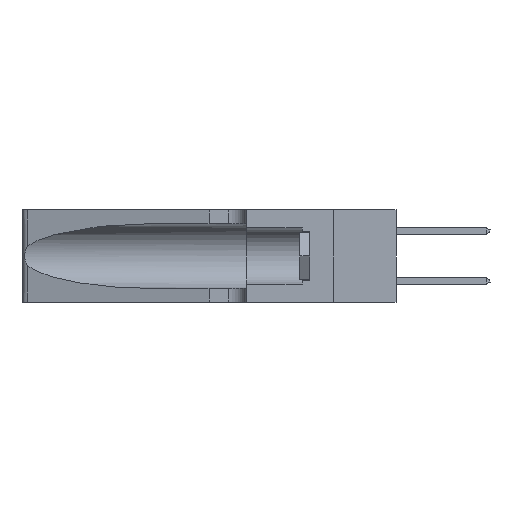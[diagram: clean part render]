
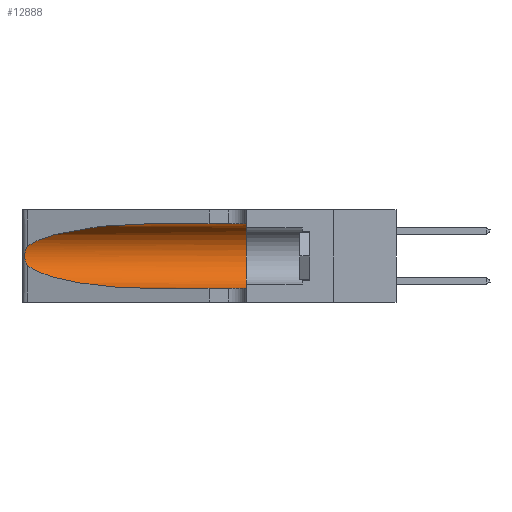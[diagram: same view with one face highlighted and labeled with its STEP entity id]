
A CAD part, left-side view. The second image highlights one B-rep face of the part: STEP entity #12888.
In plain terms, the highlighted cylindrical face has radius 3.308 mm (diameter 6.617 mm), a partial arc.
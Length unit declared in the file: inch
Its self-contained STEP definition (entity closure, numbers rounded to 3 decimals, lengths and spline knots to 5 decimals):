
#367 = AXIS2_PLACEMENT_3D ( 'NONE', #13925, #20824, #4595 ) ;
#371 = VECTOR ( 'NONE', #41196, 39.37008 ) ;
#672 = ORIENTED_EDGE ( 'NONE', *, *, #19827, .T. ) ;
#911 = EDGE_CURVE ( 'NONE', #10256, #2713, #16046, .T. ) ;
#2713 = VERTEX_POINT ( 'NONE', #16125 ) ;
#3072 = CARTESIAN_POINT ( 'NONE',  ( 0.1305, 0.72297, 0.05475 ) ) ;
#3941 = ORIENTED_EDGE ( 'NONE', *, *, #911, .T. ) ;
#4567 = ORIENTED_EDGE ( 'NONE', *, *, #37040, .F. ) ;
#4595 = DIRECTION ( 'NONE',  ( 0., 0., -1. ) ) ;
#4882 = EDGE_LOOP ( 'NONE', ( #3941, #5459, #18689, #672, #32037, #4567 ) ) ;
#4992 = VERTEX_POINT ( 'NONE', #27037 ) ;
#5459 = ORIENTED_EDGE ( 'NONE', *, *, #25994, .T. ) ;
#6293 = B_SPLINE_CURVE_WITH_KNOTS ( 'NONE', 3,
 ( #39427, #39988, #39561, #7451, #26863, #36609, #39838, #23754, #27011, #7735, #30260, #10958, #8375, #18431 ),
 .UNSPECIFIED., .F., .F.,
 ( 4, 2, 2, 2, 2, 2, 4 ),
 ( 0., 0.00027, 0.00053, 0.00107, 0.0016, 0.00187, 0.00214 ),
 .UNSPECIFIED. ) ;
#6308 = DIRECTION ( 'NONE',  ( 0., 0., 1. ) ) ;
#6640 = CARTESIAN_POINT ( 'NONE',  ( 0.1305, 1.61858, 0.05475 ) ) ;
#7451 = CARTESIAN_POINT ( 'NONE',  ( 0.25787, 1.23484, 0.2124 ) ) ;
#7735 = CARTESIAN_POINT ( 'NONE',  ( 0.25856, 1.23593, 0.16098 ) ) ;
#7917 = LINE ( 'NONE', #16062, #371 ) ;
#8375 = CARTESIAN_POINT ( 'NONE',  ( 0.25555, 1.22993, 0.14849 ) ) ;
#9449 = CARTESIAN_POINT ( 'NONE',  ( 0.25487, 1.22718, 0.22369 ) ) ;
#10256 = VERTEX_POINT ( 'NONE', #37038 ) ;
#10655 = LINE ( 'NONE', #6640, #35347 ) ;
#10958 = CARTESIAN_POINT ( 'NONE',  ( 0.25639, 1.23186, 0.15144 ) ) ;
#12888 = ADVANCED_FACE ( 'NONE', ( #35625 ), #24405, .F. ) ;
#13925 = CARTESIAN_POINT ( 'NONE',  ( 0.1305, 1.61858, 0.185 ) ) ;
#14921 = CARTESIAN_POINT ( 'NONE',  ( 0.2373, 1.15595, 0.08982 ) ) ;
#16046 =( BOUNDED_CURVE ( )  B_SPLINE_CURVE ( 3, ( #25490, #28721, #22382, #9449 ),
 .UNSPECIFIED., .F., .F. ) 
 B_SPLINE_CURVE_WITH_KNOTS ( ( 4, 4 ),
 ( 1.5708, 2.84003 ),
 .UNSPECIFIED. ) 
 CURVE ( )  GEOMETRIC_REPRESENTATION_ITEM ( )  RATIONAL_B_SPLINE_CURVE ( ( 1., 0.87, 0.87, 1. ) ) 
 REPRESENTATION_ITEM ( '' )  );
#16062 = CARTESIAN_POINT ( 'NONE',  ( 0.1305, 1.61858, 0.31525 ) ) ;
#16125 = CARTESIAN_POINT ( 'NONE',  ( 0.25487, 1.22718, 0.22369 ) ) ;
#18431 = CARTESIAN_POINT ( 'NONE',  ( 0.25487, 1.22718, 0.14631 ) ) ;
#18689 = ORIENTED_EDGE ( 'NONE', *, *, #37504, .T. ) ;
#19827 = EDGE_CURVE ( 'NONE', #23055, #23074, #10655, .T. ) ;
#20824 = DIRECTION ( 'NONE',  ( 0., -1., 0. ) ) ;
#22121 = CARTESIAN_POINT ( 'NONE',  ( 0.1305, 0.35, 0.05475 ) ) ;
#22382 = CARTESIAN_POINT ( 'NONE',  ( 0.2373, 1.15595, 0.28018 ) ) ;
#23055 = VERTEX_POINT ( 'NONE', #3072 ) ;
#23074 = VERTEX_POINT ( 'NONE', #22121 ) ;
#23754 = CARTESIAN_POINT ( 'NONE',  ( 0.26075, 1.23896, 0.178 ) ) ;
#24405 = CYLINDRICAL_SURFACE ( 'NONE', #367, 0.13025 ) ;
#25424 = DIRECTION ( 'NONE',  ( 0., 1., 0. ) ) ;
#25490 = CARTESIAN_POINT ( 'NONE',  ( 0.1305, 0.72297, 0.31525 ) ) ;
#25994 = EDGE_CURVE ( 'NONE', #2713, #4992, #6293, .T. ) ;
#26863 = CARTESIAN_POINT ( 'NONE',  ( 0.25854, 1.2359, 0.20912 ) ) ;
#27011 = CARTESIAN_POINT ( 'NONE',  ( 0.26017, 1.23833, 0.17102 ) ) ;
#27037 = CARTESIAN_POINT ( 'NONE',  ( 0.25487, 1.22718, 0.14631 ) ) ;
#27655 = CARTESIAN_POINT ( 'NONE',  ( 0.1305, 0.35, 0.31525 ) ) ;
#28721 = CARTESIAN_POINT ( 'NONE',  ( 0.18966, 0.96281, 0.31525 ) ) ;
#30260 = CARTESIAN_POINT ( 'NONE',  ( 0.25789, 1.23486, 0.15765 ) ) ;
#31844 =( BOUNDED_CURVE ( )  B_SPLINE_CURVE ( 3, ( #34235, #14921, #40038, #34099 ),
 .UNSPECIFIED., .F., .F. ) 
 B_SPLINE_CURVE_WITH_KNOTS ( ( 4, 4 ),
 ( 3.44316, 4.71239 ),
 .UNSPECIFIED. ) 
 CURVE ( )  GEOMETRIC_REPRESENTATION_ITEM ( )  RATIONAL_B_SPLINE_CURVE ( ( 1., 0.87, 0.87, 1. ) ) 
 REPRESENTATION_ITEM ( '' )  );
#32037 = ORIENTED_EDGE ( 'NONE', *, *, #35340, .F. ) ;
#34099 = CARTESIAN_POINT ( 'NONE',  ( 0.1305, 0.72297, 0.05475 ) ) ;
#34235 = CARTESIAN_POINT ( 'NONE',  ( 0.25487, 1.22718, 0.14631 ) ) ;
#35340 = EDGE_CURVE ( 'NONE', #36900, #23074, #37733, .T. ) ;
#35347 = VECTOR ( 'NONE', #37013, 39.37008 ) ;
#35625 = FACE_OUTER_BOUND ( 'NONE', #4882, .T. ) ;
#36609 = CARTESIAN_POINT ( 'NONE',  ( 0.26018, 1.23835, 0.19895 ) ) ;
#36900 = VERTEX_POINT ( 'NONE', #27655 ) ;
#37013 = DIRECTION ( 'NONE',  ( 0., -1., 0. ) ) ;
#37038 = CARTESIAN_POINT ( 'NONE',  ( 0.1305, 0.72297, 0.31525 ) ) ;
#37040 = EDGE_CURVE ( 'NONE', #10256, #36900, #7917, .T. ) ;
#37504 = EDGE_CURVE ( 'NONE', #4992, #23055, #31844, .T. ) ;
#37733 = CIRCLE ( 'NONE', #39121, 0.13025 ) ;
#38545 = CARTESIAN_POINT ( 'NONE',  ( 0.1305, 0.35, 0.185 ) ) ;
#39121 = AXIS2_PLACEMENT_3D ( 'NONE', #38545, #25424, #6308 ) ;
#39427 = CARTESIAN_POINT ( 'NONE',  ( 0.25487, 1.22718, 0.22369 ) ) ;
#39561 = CARTESIAN_POINT ( 'NONE',  ( 0.25639, 1.23184, 0.21858 ) ) ;
#39838 = CARTESIAN_POINT ( 'NONE',  ( 0.26075, 1.23896, 0.19203 ) ) ;
#39988 = CARTESIAN_POINT ( 'NONE',  ( 0.25555, 1.22994, 0.2215 ) ) ;
#40038 = CARTESIAN_POINT ( 'NONE',  ( 0.18966, 0.96281, 0.05475 ) ) ;
#41196 = DIRECTION ( 'NONE',  ( 0., -1., 0. ) ) ;
